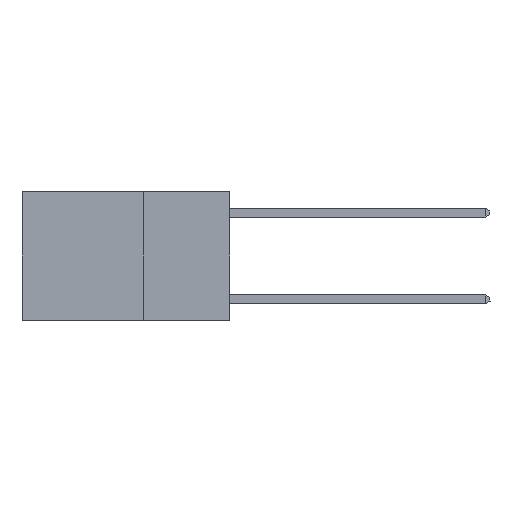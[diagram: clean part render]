
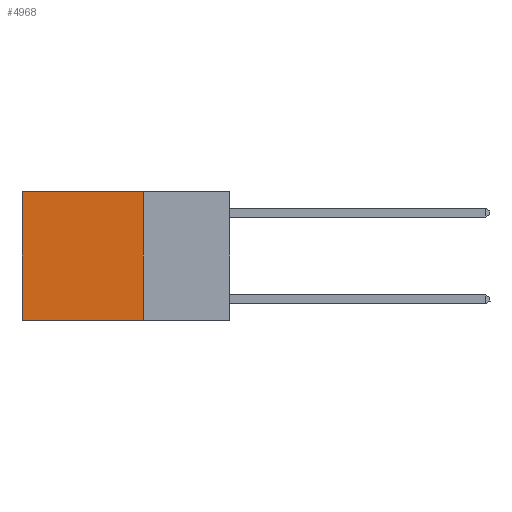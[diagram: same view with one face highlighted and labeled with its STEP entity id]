
A CAD part, left-side view. The second image highlights one B-rep face of the part: STEP entity #4968.
In plain terms, the highlighted planar face has unit normal (-1, 0, 0).
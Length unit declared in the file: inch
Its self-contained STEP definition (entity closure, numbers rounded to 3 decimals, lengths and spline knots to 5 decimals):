
#516 = EDGE_CURVE ( 'NONE', #1760, #5008, #3289, .T. ) ;
#628 = LINE ( 'NONE', #4947, #3039 ) ;
#1151 = LINE ( 'NONE', #10054, #8946 ) ;
#1760 = VERTEX_POINT ( 'NONE', #11215 ) ;
#2036 = EDGE_LOOP ( 'NONE', ( #10356, #14805, #13193, #11717 ) ) ;
#2078 = DIRECTION ( 'NONE',  ( 1., 0., 0. ) ) ;
#2741 = LINE ( 'NONE', #3392, #4331 ) ;
#3039 = VECTOR ( 'NONE', #15185, 39.37008 ) ;
#3251 = DIRECTION ( 'NONE',  ( 0., 0., -1. ) ) ;
#3289 = LINE ( 'NONE', #10382, #6288 ) ;
#3392 = CARTESIAN_POINT ( 'NONE',  ( 0.2625, 0.25, 0. ) ) ;
#3412 = DIRECTION ( 'NONE',  ( 0., 1., 0. ) ) ;
#4185 = AXIS2_PLACEMENT_3D ( 'NONE', #9562, #2078, #3251 ) ;
#4331 = VECTOR ( 'NONE', #5797, 39.37008 ) ;
#4947 = CARTESIAN_POINT ( 'NONE',  ( 0.2625, 0.6, 0. ) ) ;
#4968 = ADVANCED_FACE ( 'NONE', ( #6748 ), #6781, .F. ) ;
#5008 = VERTEX_POINT ( 'NONE', #9790 ) ;
#5748 = VERTEX_POINT ( 'NONE', #14739 ) ;
#5797 = DIRECTION ( 'NONE',  ( 0., 0., -1. ) ) ;
#6279 = VERTEX_POINT ( 'NONE', #14657 ) ;
#6288 = VECTOR ( 'NONE', #11662, 39.37008 ) ;
#6748 = FACE_OUTER_BOUND ( 'NONE', #2036, .T. ) ;
#6781 = PLANE ( 'NONE',  #4185 ) ;
#8946 = VECTOR ( 'NONE', #3412, 39.37008 ) ;
#9562 = CARTESIAN_POINT ( 'NONE',  ( 0.2625, 0.25, 0. ) ) ;
#9790 = CARTESIAN_POINT ( 'NONE',  ( 0.2625, 0.6, -0.37 ) ) ;
#10054 = CARTESIAN_POINT ( 'NONE',  ( 0.2625, 0.25, 0. ) ) ;
#10356 = ORIENTED_EDGE ( 'NONE', *, *, #15728, .T. ) ;
#10382 = CARTESIAN_POINT ( 'NONE',  ( 0.2625, 0.25, -0.37 ) ) ;
#10398 = EDGE_CURVE ( 'NONE', #5748, #6279, #1151, .T. ) ;
#11003 = EDGE_CURVE ( 'NONE', #5748, #1760, #2741, .T. ) ;
#11215 = CARTESIAN_POINT ( 'NONE',  ( 0.2625, 0.25, -0.37 ) ) ;
#11662 = DIRECTION ( 'NONE',  ( 0., 1., 0. ) ) ;
#11717 = ORIENTED_EDGE ( 'NONE', *, *, #10398, .T. ) ;
#13193 = ORIENTED_EDGE ( 'NONE', *, *, #11003, .F. ) ;
#14657 = CARTESIAN_POINT ( 'NONE',  ( 0.2625, 0.6, 0. ) ) ;
#14739 = CARTESIAN_POINT ( 'NONE',  ( 0.2625, 0.25, 0. ) ) ;
#14805 = ORIENTED_EDGE ( 'NONE', *, *, #516, .F. ) ;
#15185 = DIRECTION ( 'NONE',  ( 0., 0., -1. ) ) ;
#15728 = EDGE_CURVE ( 'NONE', #6279, #5008, #628, .T. ) ;
